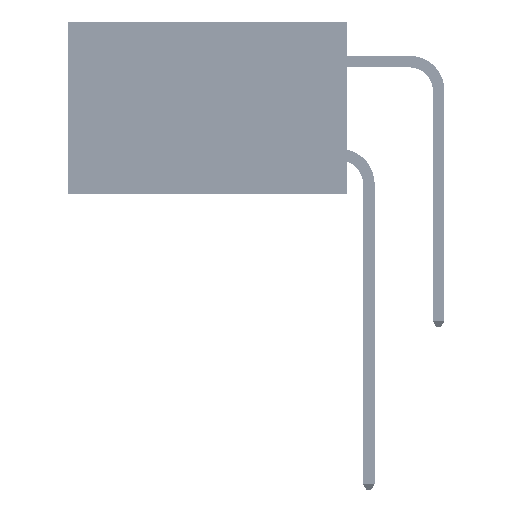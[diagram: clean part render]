
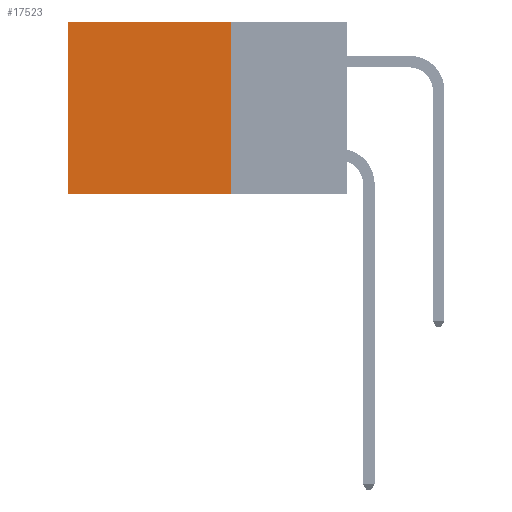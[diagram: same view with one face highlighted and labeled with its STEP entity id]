
A CAD part, left-side view. The second image highlights one B-rep face of the part: STEP entity #17523.
In plain terms, the highlighted planar face has unit normal (-1, 0, 0).
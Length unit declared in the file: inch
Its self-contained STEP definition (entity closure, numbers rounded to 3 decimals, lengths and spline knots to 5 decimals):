
#19 = DIRECTION ( 'NONE',  ( 1., 0., 0. ) ) ;
#117 = EDGE_CURVE ( 'NONE', #34946, #46609, #41748, .T. ) ;
#1187 = CARTESIAN_POINT ( 'NONE',  ( 0.2875, 0.6, -0.37 ) ) ;
#1412 = CARTESIAN_POINT ( 'NONE',  ( 0.2875, 0.25, -0.37 ) ) ;
#1633 = DIRECTION ( 'NONE',  ( 0., 0., -1. ) ) ;
#2088 = FACE_OUTER_BOUND ( 'NONE', #8531, .T. ) ;
#4261 = PLANE ( 'NONE',  #42456 ) ;
#5135 = CARTESIAN_POINT ( 'NONE',  ( 0.2875, 0.25, 0. ) ) ;
#5698 = ORIENTED_EDGE ( 'NONE', *, *, #34218, .F. ) ;
#6160 = ORIENTED_EDGE ( 'NONE', *, *, #38368, .T. ) ;
#7560 = CARTESIAN_POINT ( 'NONE',  ( 0.2875, 0.25, 0. ) ) ;
#8531 = EDGE_LOOP ( 'NONE', ( #38922, #5698, #37405, #6160 ) ) ;
#8832 = DIRECTION ( 'NONE',  ( 0., 1., 0. ) ) ;
#9115 = VECTOR ( 'NONE', #1633, 39.37008 ) ;
#14302 = EDGE_CURVE ( 'NONE', #40308, #22815, #31194, .T. ) ;
#14870 = VECTOR ( 'NONE', #45888, 39.37008 ) ;
#17402 = CARTESIAN_POINT ( 'NONE',  ( 0.2875, 0.25, 0. ) ) ;
#17523 = ADVANCED_FACE ( 'NONE', ( #2088 ), #4261, .F. ) ;
#22815 = VERTEX_POINT ( 'NONE', #1412 ) ;
#22989 = LINE ( 'NONE', #37555, #43394 ) ;
#26147 = DIRECTION ( 'NONE',  ( 0., 0., -1. ) ) ;
#27576 = CARTESIAN_POINT ( 'NONE',  ( 0.2875, 0.6, 0. ) ) ;
#31194 = LINE ( 'NONE', #5135, #14870 ) ;
#34218 = EDGE_CURVE ( 'NONE', #22815, #46609, #22989, .T. ) ;
#34946 = VERTEX_POINT ( 'NONE', #37659 ) ;
#36118 = CARTESIAN_POINT ( 'NONE',  ( 0.2875, 0.25, 0. ) ) ;
#37405 = ORIENTED_EDGE ( 'NONE', *, *, #14302, .F. ) ;
#37555 = CARTESIAN_POINT ( 'NONE',  ( 0.2875, 0.25, -0.37 ) ) ;
#37659 = CARTESIAN_POINT ( 'NONE',  ( 0.2875, 0.6, 0. ) ) ;
#38368 = EDGE_CURVE ( 'NONE', #40308, #34946, #38488, .T. ) ;
#38488 = LINE ( 'NONE', #17402, #46588 ) ;
#38922 = ORIENTED_EDGE ( 'NONE', *, *, #117, .T. ) ;
#39576 = DIRECTION ( 'NONE',  ( 0., 1., 0. ) ) ;
#40308 = VERTEX_POINT ( 'NONE', #36118 ) ;
#41748 = LINE ( 'NONE', #27576, #9115 ) ;
#42456 = AXIS2_PLACEMENT_3D ( 'NONE', #7560, #19, #26147 ) ;
#43394 = VECTOR ( 'NONE', #8832, 39.37008 ) ;
#45888 = DIRECTION ( 'NONE',  ( 0., 0., -1. ) ) ;
#46588 = VECTOR ( 'NONE', #39576, 39.37008 ) ;
#46609 = VERTEX_POINT ( 'NONE', #1187 ) ;
